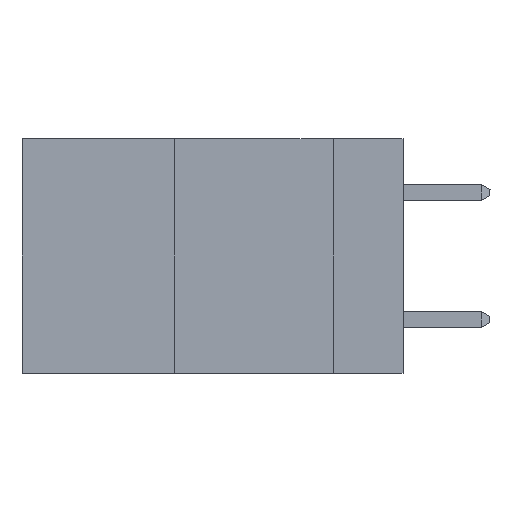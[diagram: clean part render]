
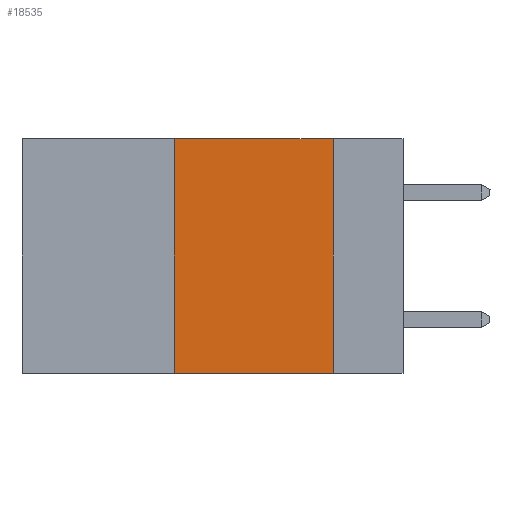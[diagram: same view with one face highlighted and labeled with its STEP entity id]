
A CAD part, left-side view. The second image highlights one B-rep face of the part: STEP entity #18535.
In plain terms, the highlighted planar face has unit normal (-1, 0, 0).
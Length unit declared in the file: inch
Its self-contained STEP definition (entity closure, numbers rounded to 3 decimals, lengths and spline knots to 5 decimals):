
#748 = EDGE_CURVE ( 'NONE', #11510, #9752, #8697, .T. ) ;
#1247 = CARTESIAN_POINT ( 'NONE',  ( 0., 0.6, 0. ) ) ;
#1317 = VECTOR ( 'NONE', #21016, 39.37008 ) ;
#1448 = ORIENTED_EDGE ( 'NONE', *, *, #748, .T. ) ;
#2038 = VECTOR ( 'NONE', #15709, 39.37008 ) ;
#2471 = DIRECTION ( 'NONE',  ( 0., -1., 0. ) ) ;
#2647 = EDGE_CURVE ( 'NONE', #11510, #5788, #7098, .T. ) ;
#4377 = EDGE_CURVE ( 'NONE', #12810, #9752, #14504, .T. ) ;
#4738 = CARTESIAN_POINT ( 'NONE',  ( 0., 0.11, 0. ) ) ;
#4854 = AXIS2_PLACEMENT_3D ( 'NONE', #19744, #11278, #16405 ) ;
#5453 = CARTESIAN_POINT ( 'NONE',  ( 0., 0.36, -0.37 ) ) ;
#5779 = ORIENTED_EDGE ( 'NONE', *, *, #2647, .F. ) ;
#5788 = VERTEX_POINT ( 'NONE', #6170 ) ;
#6170 = CARTESIAN_POINT ( 'NONE',  ( 0., 0.36, 0. ) ) ;
#6776 = LINE ( 'NONE', #1247, #1317 ) ;
#7098 = LINE ( 'NONE', #12490, #17472 ) ;
#8329 = ORIENTED_EDGE ( 'NONE', *, *, #4377, .F. ) ;
#8697 = LINE ( 'NONE', #10726, #18550 ) ;
#9752 = VERTEX_POINT ( 'NONE', #10150 ) ;
#10150 = CARTESIAN_POINT ( 'NONE',  ( 0., 0.11, -0.37 ) ) ;
#10726 = CARTESIAN_POINT ( 'NONE',  ( 0., 0.6, -0.37 ) ) ;
#11278 = DIRECTION ( 'NONE',  ( 1., 0., 0. ) ) ;
#11510 = VERTEX_POINT ( 'NONE', #5453 ) ;
#12490 = CARTESIAN_POINT ( 'NONE',  ( 0., 0.36, 0. ) ) ;
#12810 = VERTEX_POINT ( 'NONE', #4738 ) ;
#13687 = ORIENTED_EDGE ( 'NONE', *, *, #19916, .F. ) ;
#14504 = LINE ( 'NONE', #16858, #2038 ) ;
#15709 = DIRECTION ( 'NONE',  ( 0., 0., -1. ) ) ;
#16405 = DIRECTION ( 'NONE',  ( 0., 0., -1. ) ) ;
#16516 = FACE_OUTER_BOUND ( 'NONE', #19574, .T. ) ;
#16858 = CARTESIAN_POINT ( 'NONE',  ( 0., 0.11, 0. ) ) ;
#17426 = DIRECTION ( 'NONE',  ( 0., 0., 1. ) ) ;
#17472 = VECTOR ( 'NONE', #17426, 39.37008 ) ;
#17753 = PLANE ( 'NONE',  #4854 ) ;
#18535 = ADVANCED_FACE ( 'NONE', ( #16516 ), #17753, .F. ) ;
#18550 = VECTOR ( 'NONE', #2471, 39.37008 ) ;
#19574 = EDGE_LOOP ( 'NONE', ( #8329, #13687, #5779, #1448 ) ) ;
#19744 = CARTESIAN_POINT ( 'NONE',  ( 0., 0.6, 0. ) ) ;
#19916 = EDGE_CURVE ( 'NONE', #5788, #12810, #6776, .T. ) ;
#21016 = DIRECTION ( 'NONE',  ( 0., -1., 0. ) ) ;
